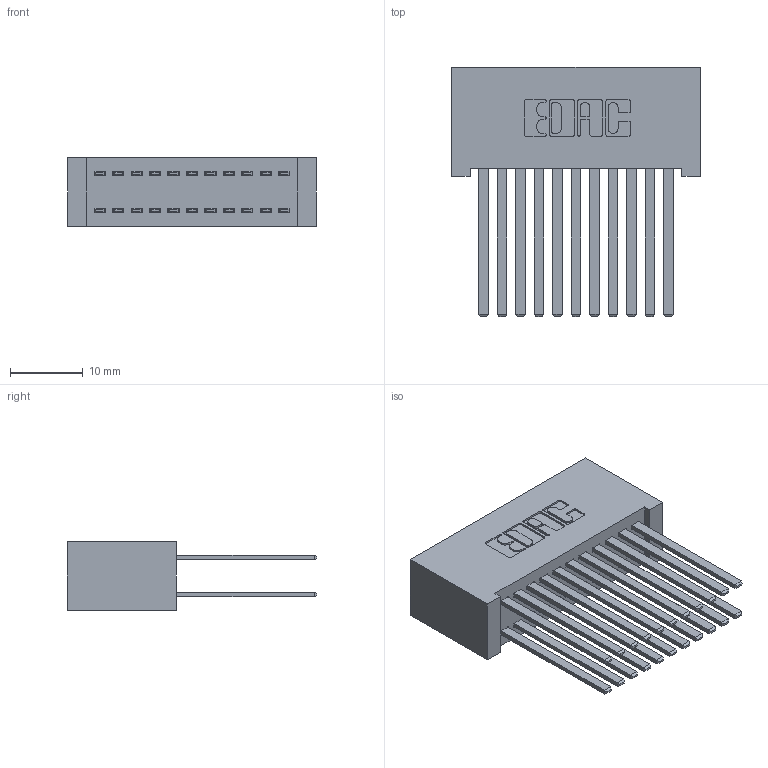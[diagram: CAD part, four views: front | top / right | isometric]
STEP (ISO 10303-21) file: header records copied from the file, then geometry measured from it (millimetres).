
FILE_DESCRIPTION (( 'STEP AP203' ), '1' );
FILE_NAME ('342-022-544-201.STEP', '2019-10-01T22:39:54', ( '' ), ( '' ), 'SwSTEP 2.0', 'SolidWorks 2016', '' );
FILE_SCHEMA (( 'CONFIG_CONTROL_DESIGN' ));
Length unit declared in the file: inch
Products named in the file (3): 342 Part_Lugless; 345-292-001_345-293-144; 342-022-544-201
Assembly tree (23 placements, depth 2):
  342-022-544-201
    342 Part_Lugless
    345-292-001_345-293-144  x22
Bounding box: 34.19 x 34.3 x 9.4 mm (x, y, z)
Volume: 3673 mm3; surface area: 6515.2 mm2
Topology: 23 solids, 23 shells, 1114 faces, 3289 edges, 2162 vertices
Faces by surface type: plane 766, cylinder 348
Entity records: 10493 total; most frequent: CARTESIAN_POINT 1770, ORIENTED_EDGE 1706, DIRECTION 1557, EDGE_CURVE 853, VECTOR 737, LINE 737, VERTEX_POINT 566, AXIS2_PLACEMENT_3D 410
